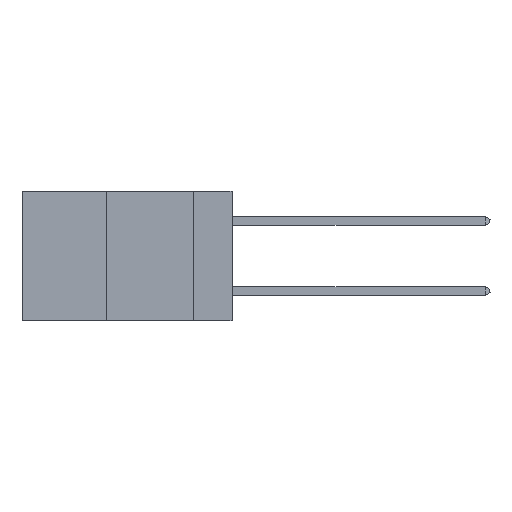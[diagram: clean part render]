
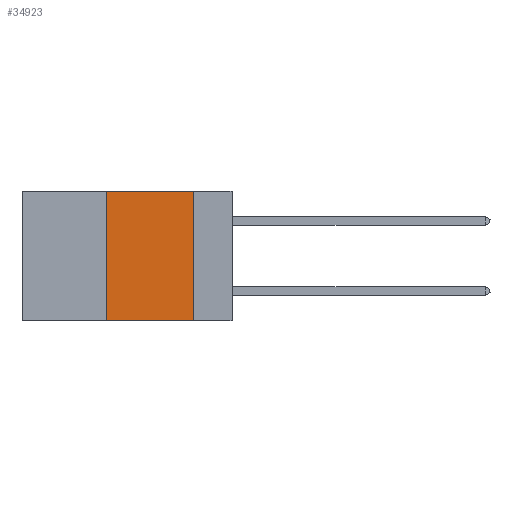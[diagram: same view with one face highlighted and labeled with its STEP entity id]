
A CAD part, left-side view. The second image highlights one B-rep face of the part: STEP entity #34923.
In plain terms, the highlighted planar face has unit normal (-1, 0, 0).
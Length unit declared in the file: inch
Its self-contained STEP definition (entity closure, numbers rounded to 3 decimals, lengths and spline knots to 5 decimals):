
#94 = EDGE_LOOP ( 'NONE', ( #2388, #4576, #14585, #26223 ) ) ;
#797 = VECTOR ( 'NONE', #28872, 39.37008 ) ;
#1534 = VECTOR ( 'NONE', #16377, 39.37008 ) ;
#2000 = VERTEX_POINT ( 'NONE', #24573 ) ;
#2388 = ORIENTED_EDGE ( 'NONE', *, *, #20476, .F. ) ;
#2638 = CARTESIAN_POINT ( 'NONE',  ( 0., 0.6, 0. ) ) ;
#2875 = LINE ( 'NONE', #5812, #33458 ) ;
#4576 = ORIENTED_EDGE ( 'NONE', *, *, #5372, .F. ) ;
#5372 = EDGE_CURVE ( 'NONE', #2000, #31110, #12218, .T. ) ;
#5812 = CARTESIAN_POINT ( 'NONE',  ( 0., 0.6, -0.37 ) ) ;
#7407 = CARTESIAN_POINT ( 'NONE',  ( 0., 0.11, -0.37 ) ) ;
#7913 = DIRECTION ( 'NONE',  ( 0., -1., 0. ) ) ;
#8675 = FACE_OUTER_BOUND ( 'NONE', #94, .T. ) ;
#8902 = LINE ( 'NONE', #32425, #1534 ) ;
#11042 = AXIS2_PLACEMENT_3D ( 'NONE', #2638, #22239, #30631 ) ;
#11963 = CARTESIAN_POINT ( 'NONE',  ( 0., 0.6, 0. ) ) ;
#12218 = LINE ( 'NONE', #11963, #797 ) ;
#14585 = ORIENTED_EDGE ( 'NONE', *, *, #22405, .F. ) ;
#16377 = DIRECTION ( 'NONE',  ( 0., 0., 1. ) ) ;
#17269 = CARTESIAN_POINT ( 'NONE',  ( 0., 0.36, -0.37 ) ) ;
#18744 = VERTEX_POINT ( 'NONE', #7407 ) ;
#20476 = EDGE_CURVE ( 'NONE', #31110, #18744, #21375, .T. ) ;
#21375 = LINE ( 'NONE', #35929, #33958 ) ;
#21759 = EDGE_CURVE ( 'NONE', #32459, #18744, #2875, .T. ) ;
#21838 = DIRECTION ( 'NONE',  ( 0., 0., -1. ) ) ;
#22239 = DIRECTION ( 'NONE',  ( 1., 0., 0. ) ) ;
#22405 = EDGE_CURVE ( 'NONE', #32459, #2000, #8902, .T. ) ;
#24573 = CARTESIAN_POINT ( 'NONE',  ( 0., 0.36, 0. ) ) ;
#25213 = PLANE ( 'NONE',  #11042 ) ;
#26223 = ORIENTED_EDGE ( 'NONE', *, *, #21759, .T. ) ;
#28872 = DIRECTION ( 'NONE',  ( 0., -1., 0. ) ) ;
#30358 = CARTESIAN_POINT ( 'NONE',  ( 0., 0.11, 0. ) ) ;
#30631 = DIRECTION ( 'NONE',  ( 0., 0., -1. ) ) ;
#31110 = VERTEX_POINT ( 'NONE', #30358 ) ;
#32425 = CARTESIAN_POINT ( 'NONE',  ( 0., 0.36, 0. ) ) ;
#32459 = VERTEX_POINT ( 'NONE', #17269 ) ;
#33458 = VECTOR ( 'NONE', #7913, 39.37008 ) ;
#33958 = VECTOR ( 'NONE', #21838, 39.37008 ) ;
#34923 = ADVANCED_FACE ( 'NONE', ( #8675 ), #25213, .F. ) ;
#35929 = CARTESIAN_POINT ( 'NONE',  ( 0., 0.11, 0. ) ) ;
